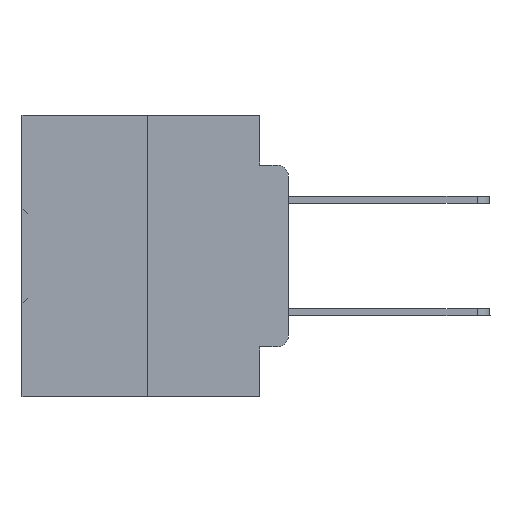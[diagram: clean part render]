
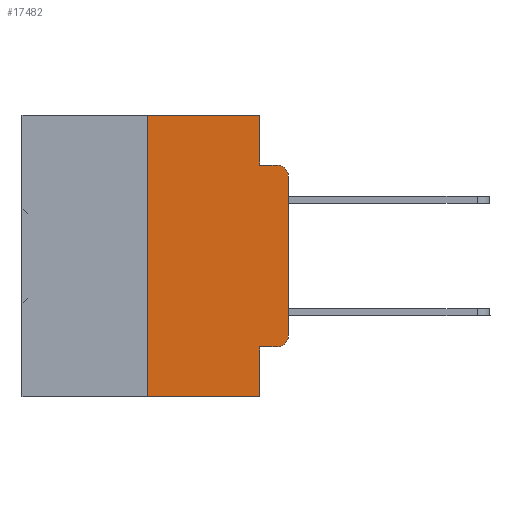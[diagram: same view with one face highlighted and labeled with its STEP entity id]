
A CAD part, left-side view. The second image highlights one B-rep face of the part: STEP entity #17482.
In plain terms, the highlighted planar face has unit normal (-1, 0, 0).
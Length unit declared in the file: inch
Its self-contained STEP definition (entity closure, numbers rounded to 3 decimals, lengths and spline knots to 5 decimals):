
#1470 = DIRECTION ( 'NONE',  ( 0., -1., 0. ) ) ;
#1535 = EDGE_CURVE ( 'NONE', #29804, #29440, #9804, .T. ) ;
#3039 = ORIENTED_EDGE ( 'NONE', *, *, #6707, .F. ) ;
#3233 = CARTESIAN_POINT ( 'NONE',  ( 0., 0.051, -0.4115 ) ) ;
#3308 = EDGE_CURVE ( 'NONE', #19968, #9956, #30824, .T. ) ;
#3384 = VERTEX_POINT ( 'NONE', #3233 ) ;
#3593 = EDGE_CURVE ( 'NONE', #3384, #36251, #34004, .T. ) ;
#4188 = VERTEX_POINT ( 'NONE', #28035 ) ;
#5569 = VECTOR ( 'NONE', #29442, 39.37008 ) ;
#5937 = CARTESIAN_POINT ( 'NONE',  ( 0., 0.051, -0.0885 ) ) ;
#6052 = ORIENTED_EDGE ( 'NONE', *, *, #21300, .T. ) ;
#6086 = DIRECTION ( 'NONE',  ( 0., 0., -1. ) ) ;
#6303 = VERTEX_POINT ( 'NONE', #9683 ) ;
#6463 = VECTOR ( 'NONE', #32107, 39.37008 ) ;
#6707 = EDGE_CURVE ( 'NONE', #3384, #4188, #33556, .T. ) ;
#6717 = LINE ( 'NONE', #16202, #26530 ) ;
#6850 = ORIENTED_EDGE ( 'NONE', *, *, #1535, .F. ) ;
#7134 = AXIS2_PLACEMENT_3D ( 'NONE', #29635, #16564, #18067 ) ;
#8295 = CARTESIAN_POINT ( 'NONE',  ( 0., 0.473, 0. ) ) ;
#8701 = ORIENTED_EDGE ( 'NONE', *, *, #35760, .T. ) ;
#8819 = VECTOR ( 'NONE', #15723, 39.37008 ) ;
#9038 = CARTESIAN_POINT ( 'NONE',  ( 0., 0.02, -0.1085 ) ) ;
#9680 = LINE ( 'NONE', #26464, #6463 ) ;
#9683 = CARTESIAN_POINT ( 'NONE',  ( 0., 0.051, -0.0885 ) ) ;
#9804 = LINE ( 'NONE', #28390, #14850 ) ;
#9956 = VERTEX_POINT ( 'NONE', #23489 ) ;
#10566 = VECTOR ( 'NONE', #34814, 39.37008 ) ;
#12001 = DIRECTION ( 'NONE',  ( -1., 0., 0. ) ) ;
#12229 = ORIENTED_EDGE ( 'NONE', *, *, #15741, .F. ) ;
#12401 = ORIENTED_EDGE ( 'NONE', *, *, #34578, .F. ) ;
#12766 = CARTESIAN_POINT ( 'NONE',  ( 0., 0., 0. ) ) ;
#13859 = CARTESIAN_POINT ( 'NONE',  ( 0., 0.051, 0. ) ) ;
#14253 = AXIS2_PLACEMENT_3D ( 'NONE', #9038, #12001, #6086 ) ;
#14850 = VECTOR ( 'NONE', #30937, 39.37008 ) ;
#15723 = DIRECTION ( 'NONE',  ( 0., 0., 1. ) ) ;
#15741 = EDGE_CURVE ( 'NONE', #22451, #6303, #34563, .T. ) ;
#16202 = CARTESIAN_POINT ( 'NONE',  ( 0., 0.473, -0.5 ) ) ;
#16403 = CARTESIAN_POINT ( 'NONE',  ( 0., 0., -0.1085 ) ) ;
#16564 = DIRECTION ( 'NONE',  ( -1., 0., 0. ) ) ;
#16679 = PLANE ( 'NONE',  #28976 ) ;
#17482 = ADVANCED_FACE ( 'NONE', ( #21047 ), #16679, .F. ) ;
#18067 = DIRECTION ( 'NONE',  ( 0., 0., -1. ) ) ;
#18566 = ORIENTED_EDGE ( 'NONE', *, *, #21493, .F. ) ;
#18765 = CARTESIAN_POINT ( 'NONE',  ( 0., 0.051, 0. ) ) ;
#18854 = VECTOR ( 'NONE', #31487, 39.37008 ) ;
#19125 = ORIENTED_EDGE ( 'NONE', *, *, #3593, .T. ) ;
#19682 = CARTESIAN_POINT ( 'NONE',  ( 0., 0.051, 0. ) ) ;
#19968 = VERTEX_POINT ( 'NONE', #16403 ) ;
#21047 = FACE_OUTER_BOUND ( 'NONE', #34371, .T. ) ;
#21197 = LINE ( 'NONE', #5937, #5569 ) ;
#21300 = EDGE_CURVE ( 'NONE', #28324, #19968, #22629, .T. ) ;
#21493 = EDGE_CURVE ( 'NONE', #6303, #9956, #21197, .T. ) ;
#22053 = CARTESIAN_POINT ( 'NONE',  ( 0., 0., -0.3915 ) ) ;
#22451 = VERTEX_POINT ( 'NONE', #13859 ) ;
#22590 = DIRECTION ( 'NONE',  ( 1., 0., 0. ) ) ;
#22629 = LINE ( 'NONE', #12766, #8819 ) ;
#23489 = CARTESIAN_POINT ( 'NONE',  ( 0., 0.02, -0.0885 ) ) ;
#24154 = CARTESIAN_POINT ( 'NONE',  ( 0., 0.25, 0. ) ) ;
#25533 = EDGE_CURVE ( 'NONE', #29804, #4188, #6717, .T. ) ;
#26464 = CARTESIAN_POINT ( 'NONE',  ( 0., 0.473, 0. ) ) ;
#26530 = VECTOR ( 'NONE', #1470, 39.37008 ) ;
#28035 = CARTESIAN_POINT ( 'NONE',  ( 0., 0.051, -0.5 ) ) ;
#28324 = VERTEX_POINT ( 'NONE', #22053 ) ;
#28390 = CARTESIAN_POINT ( 'NONE',  ( 0., 0.25, 0. ) ) ;
#28539 = CARTESIAN_POINT ( 'NONE',  ( 0., 0.051, -0.4115 ) ) ;
#28622 = VECTOR ( 'NONE', #37369, 39.37008 ) ;
#28765 = CARTESIAN_POINT ( 'NONE',  ( 0., 0.25, -0.5 ) ) ;
#28976 = AXIS2_PLACEMENT_3D ( 'NONE', #8295, #22590, #37204 ) ;
#29440 = VERTEX_POINT ( 'NONE', #24154 ) ;
#29442 = DIRECTION ( 'NONE',  ( 0., -1., 0. ) ) ;
#29635 = CARTESIAN_POINT ( 'NONE',  ( 0., 0.02, -0.3915 ) ) ;
#29804 = VERTEX_POINT ( 'NONE', #28765 ) ;
#30655 = ORIENTED_EDGE ( 'NONE', *, *, #3308, .T. ) ;
#30824 = CIRCLE ( 'NONE', #14253, 0.02 ) ;
#30937 = DIRECTION ( 'NONE',  ( 0., 0., 1. ) ) ;
#31487 = DIRECTION ( 'NONE',  ( 0., -1., 0. ) ) ;
#32107 = DIRECTION ( 'NONE',  ( 0., -1., 0. ) ) ;
#32571 = CARTESIAN_POINT ( 'NONE',  ( 0., 0.02, -0.4115 ) ) ;
#33556 = LINE ( 'NONE', #18765, #10566 ) ;
#34004 = LINE ( 'NONE', #28539, #18854 ) ;
#34203 = ORIENTED_EDGE ( 'NONE', *, *, #25533, .T. ) ;
#34371 = EDGE_LOOP ( 'NONE', ( #6052, #30655, #18566, #12229, #12401, #6850, #34203, #3039, #19125, #8701 ) ) ;
#34563 = LINE ( 'NONE', #19682, #28622 ) ;
#34578 = EDGE_CURVE ( 'NONE', #29440, #22451, #9680, .T. ) ;
#34814 = DIRECTION ( 'NONE',  ( 0., 0., -1. ) ) ;
#35760 = EDGE_CURVE ( 'NONE', #36251, #28324, #37206, .T. ) ;
#36251 = VERTEX_POINT ( 'NONE', #32571 ) ;
#37204 = DIRECTION ( 'NONE',  ( 0., 0., -1. ) ) ;
#37206 = CIRCLE ( 'NONE', #7134, 0.02 ) ;
#37369 = DIRECTION ( 'NONE',  ( 0., 0., -1. ) ) ;
